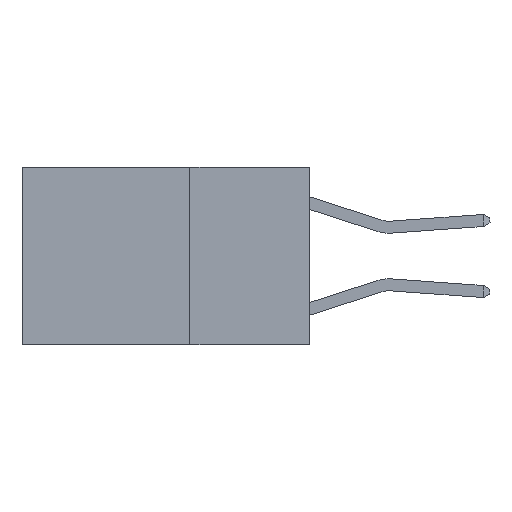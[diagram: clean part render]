
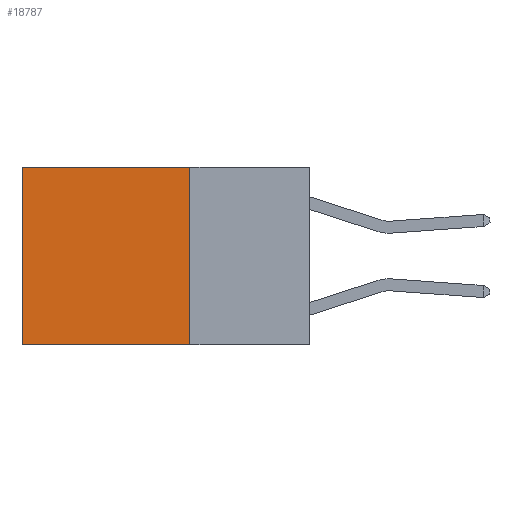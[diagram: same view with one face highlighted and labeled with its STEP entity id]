
A CAD part, left-side view. The second image highlights one B-rep face of the part: STEP entity #18787.
In plain terms, the highlighted planar face has unit normal (-1, 0, 0).
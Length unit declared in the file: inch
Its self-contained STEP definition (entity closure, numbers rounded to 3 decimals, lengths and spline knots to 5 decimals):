
#646 = AXIS2_PLACEMENT_3D ( 'NONE', #7015, #8797, #21102 ) ;
#793 = LINE ( 'NONE', #15530, #19573 ) ;
#1202 = VERTEX_POINT ( 'NONE', #9813 ) ;
#2151 = VECTOR ( 'NONE', #20444, 39.37008 ) ;
#2908 = EDGE_CURVE ( 'NONE', #7747, #1202, #17088, .T. ) ;
#2996 = ORIENTED_EDGE ( 'NONE', *, *, #2908, .F. ) ;
#4930 = VERTEX_POINT ( 'NONE', #18447 ) ;
#6463 = VECTOR ( 'NONE', #22473, 39.37008 ) ;
#7015 = CARTESIAN_POINT ( 'NONE',  ( 0.2625, 0.25, 0. ) ) ;
#7747 = VERTEX_POINT ( 'NONE', #14157 ) ;
#8222 = EDGE_LOOP ( 'NONE', ( #9015, #2996, #21053, #19536 ) ) ;
#8273 = VECTOR ( 'NONE', #22812, 39.37008 ) ;
#8746 = CARTESIAN_POINT ( 'NONE',  ( 0.2625, 0.25, -0.37 ) ) ;
#8797 = DIRECTION ( 'NONE',  ( 1., 0., 0. ) ) ;
#9015 = ORIENTED_EDGE ( 'NONE', *, *, #14416, .T. ) ;
#9813 = CARTESIAN_POINT ( 'NONE',  ( 0.2625, 0.6, -0.37 ) ) ;
#10257 = DIRECTION ( 'NONE',  ( 0., 0., -1. ) ) ;
#11163 = LINE ( 'NONE', #17178, #6463 ) ;
#11885 = EDGE_CURVE ( 'NONE', #4930, #19111, #11163, .T. ) ;
#12764 = FACE_OUTER_BOUND ( 'NONE', #8222, .T. ) ;
#14157 = CARTESIAN_POINT ( 'NONE',  ( 0.2625, 0.25, -0.37 ) ) ;
#14416 = EDGE_CURVE ( 'NONE', #19111, #1202, #793, .T. ) ;
#15530 = CARTESIAN_POINT ( 'NONE',  ( 0.2625, 0.6, 0. ) ) ;
#16185 = LINE ( 'NONE', #18695, #2151 ) ;
#17088 = LINE ( 'NONE', #8746, #8273 ) ;
#17178 = CARTESIAN_POINT ( 'NONE',  ( 0.2625, 0.25, 0. ) ) ;
#18447 = CARTESIAN_POINT ( 'NONE',  ( 0.2625, 0.25, 0. ) ) ;
#18695 = CARTESIAN_POINT ( 'NONE',  ( 0.2625, 0.25, 0. ) ) ;
#18787 = ADVANCED_FACE ( 'NONE', ( #12764 ), #19333, .F. ) ;
#19111 = VERTEX_POINT ( 'NONE', #21926 ) ;
#19333 = PLANE ( 'NONE',  #646 ) ;
#19536 = ORIENTED_EDGE ( 'NONE', *, *, #11885, .T. ) ;
#19573 = VECTOR ( 'NONE', #10257, 39.37008 ) ;
#20444 = DIRECTION ( 'NONE',  ( 0., 0., -1. ) ) ;
#21053 = ORIENTED_EDGE ( 'NONE', *, *, #21595, .F. ) ;
#21102 = DIRECTION ( 'NONE',  ( 0., 0., -1. ) ) ;
#21595 = EDGE_CURVE ( 'NONE', #4930, #7747, #16185, .T. ) ;
#21926 = CARTESIAN_POINT ( 'NONE',  ( 0.2625, 0.6, 0. ) ) ;
#22473 = DIRECTION ( 'NONE',  ( 0., 1., 0. ) ) ;
#22812 = DIRECTION ( 'NONE',  ( 0., 1., 0. ) ) ;
